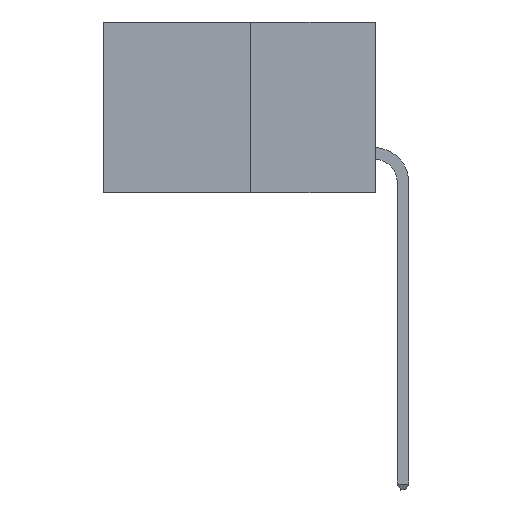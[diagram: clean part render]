
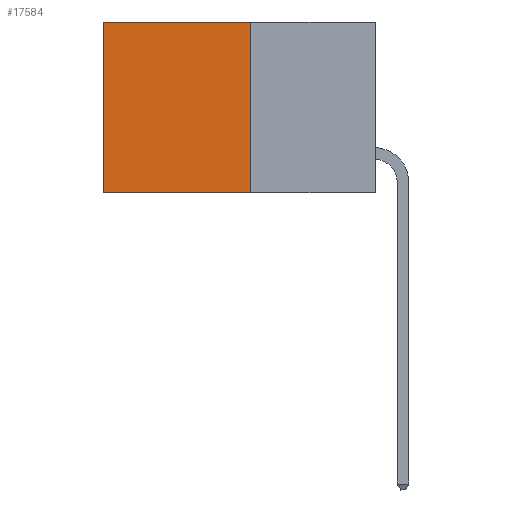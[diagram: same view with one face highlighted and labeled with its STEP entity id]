
A CAD part, left-side view. The second image highlights one B-rep face of the part: STEP entity #17584.
In plain terms, the highlighted planar face has unit normal (-1, 0, 0).
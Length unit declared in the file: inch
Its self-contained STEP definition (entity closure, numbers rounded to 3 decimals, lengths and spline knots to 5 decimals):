
#49 = CARTESIAN_POINT ( 'NONE',  ( 0.277, 0.59, 0. ) ) ;
#844 = VERTEX_POINT ( 'NONE', #14702 ) ;
#1451 = DIRECTION ( 'NONE',  ( 1., 0., 0. ) ) ;
#1607 = CARTESIAN_POINT ( 'NONE',  ( 0.277, 0.27, 0. ) ) ;
#1914 = CARTESIAN_POINT ( 'NONE',  ( 0.277, 0.27, -0.37 ) ) ;
#2498 = ORIENTED_EDGE ( 'NONE', *, *, #22003, .T. ) ;
#3077 = PLANE ( 'NONE',  #7909 ) ;
#3131 = DIRECTION ( 'NONE',  ( 0., 0., -1. ) ) ;
#3318 = VECTOR ( 'NONE', #3131, 39.37008 ) ;
#3490 = DIRECTION ( 'NONE',  ( 0., 1., 0. ) ) ;
#3943 = LINE ( 'NONE', #1607, #17860 ) ;
#4415 = ORIENTED_EDGE ( 'NONE', *, *, #22931, .T. ) ;
#5265 = VERTEX_POINT ( 'NONE', #49 ) ;
#5601 = EDGE_CURVE ( 'NONE', #23031, #844, #8234, .T. ) ;
#5883 = LINE ( 'NONE', #14776, #10223 ) ;
#7719 = VECTOR ( 'NONE', #14703, 39.37008 ) ;
#7807 = CARTESIAN_POINT ( 'NONE',  ( 0.277, 0.27, 0. ) ) ;
#7909 = AXIS2_PLACEMENT_3D ( 'NONE', #12464, #1451, #14274 ) ;
#8234 = LINE ( 'NONE', #10469, #3318 ) ;
#10223 = VECTOR ( 'NONE', #18373, 39.37008 ) ;
#10469 = CARTESIAN_POINT ( 'NONE',  ( 0.277, 0.27, -0.37 ) ) ;
#11307 = ORIENTED_EDGE ( 'NONE', *, *, #13618, .F. ) ;
#12464 = CARTESIAN_POINT ( 'NONE',  ( 0.277, 0.27, -0.37 ) ) ;
#13618 = EDGE_CURVE ( 'NONE', #844, #22813, #17347, .T. ) ;
#14274 = DIRECTION ( 'NONE',  ( 0., 0., -1. ) ) ;
#14702 = CARTESIAN_POINT ( 'NONE',  ( 0.277, 0.27, -0.37 ) ) ;
#14703 = DIRECTION ( 'NONE',  ( 0., 1., 0. ) ) ;
#14776 = CARTESIAN_POINT ( 'NONE',  ( 0.277, 0.59, -0.37 ) ) ;
#17347 = LINE ( 'NONE', #1914, #7719 ) ;
#17538 = FACE_OUTER_BOUND ( 'NONE', #22737, .T. ) ;
#17584 = ADVANCED_FACE ( 'NONE', ( #17538 ), #3077, .F. ) ;
#17751 = ORIENTED_EDGE ( 'NONE', *, *, #5601, .F. ) ;
#17860 = VECTOR ( 'NONE', #3490, 39.37008 ) ;
#18373 = DIRECTION ( 'NONE',  ( 0., 0., -1. ) ) ;
#22003 = EDGE_CURVE ( 'NONE', #23031, #5265, #3943, .T. ) ;
#22737 = EDGE_LOOP ( 'NONE', ( #4415, #11307, #17751, #2498 ) ) ;
#22813 = VERTEX_POINT ( 'NONE', #23280 ) ;
#22931 = EDGE_CURVE ( 'NONE', #5265, #22813, #5883, .T. ) ;
#23031 = VERTEX_POINT ( 'NONE', #7807 ) ;
#23280 = CARTESIAN_POINT ( 'NONE',  ( 0.277, 0.59, -0.37 ) ) ;
